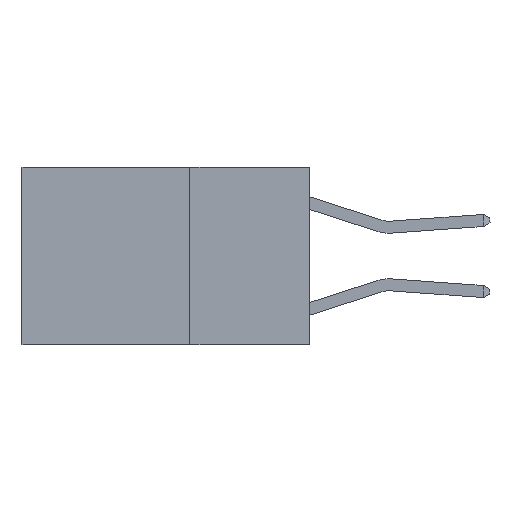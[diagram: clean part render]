
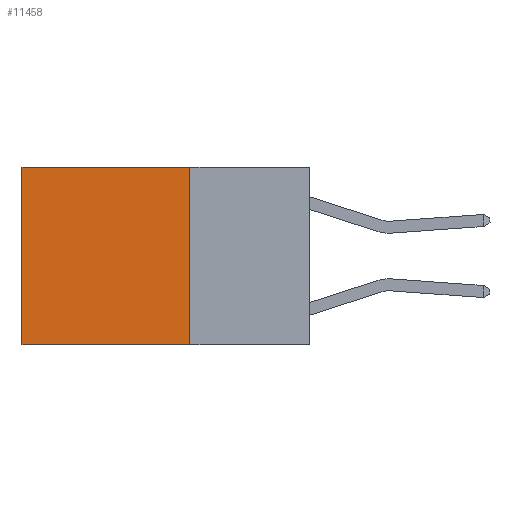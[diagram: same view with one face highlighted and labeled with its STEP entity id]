
A CAD part, left-side view. The second image highlights one B-rep face of the part: STEP entity #11458.
In plain terms, the highlighted planar face has unit normal (-1, 0, 0).
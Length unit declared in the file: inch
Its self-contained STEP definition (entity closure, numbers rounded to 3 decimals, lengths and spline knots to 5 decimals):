
#549 = DIRECTION ( 'NONE',  ( 0., 0., -1. ) ) ;
#1560 = VECTOR ( 'NONE', #18103, 39.37008 ) ;
#1615 = VERTEX_POINT ( 'NONE', #12100 ) ;
#2018 = EDGE_CURVE ( 'NONE', #11484, #3842, #4054, .T. ) ;
#2330 = LINE ( 'NONE', #20022, #9081 ) ;
#3172 = ORIENTED_EDGE ( 'NONE', *, *, #21066, .T. ) ;
#3365 = CARTESIAN_POINT ( 'NONE',  ( 0.2625, 0.25, 0. ) ) ;
#3842 = VERTEX_POINT ( 'NONE', #13780 ) ;
#4054 = LINE ( 'NONE', #11762, #20720 ) ;
#4917 = CARTESIAN_POINT ( 'NONE',  ( 0.2625, 0.25, 0. ) ) ;
#6574 = DIRECTION ( 'NONE',  ( 0., 0., -1. ) ) ;
#6920 = CARTESIAN_POINT ( 'NONE',  ( 0.2625, 0.25, 0. ) ) ;
#6943 = EDGE_CURVE ( 'NONE', #16107, #1615, #12388, .T. ) ;
#7132 = DIRECTION ( 'NONE',  ( 1., 0., 0. ) ) ;
#8471 = DIRECTION ( 'NONE',  ( 0., 1., 0. ) ) ;
#9081 = VECTOR ( 'NONE', #8471, 39.37008 ) ;
#9291 = ORIENTED_EDGE ( 'NONE', *, *, #18283, .F. ) ;
#11098 = VECTOR ( 'NONE', #6574, 39.37008 ) ;
#11458 = ADVANCED_FACE ( 'NONE', ( #20952 ), #16909, .F. ) ;
#11484 = VERTEX_POINT ( 'NONE', #15468 ) ;
#11762 = CARTESIAN_POINT ( 'NONE',  ( 0.2625, 0.6, 0. ) ) ;
#12100 = CARTESIAN_POINT ( 'NONE',  ( 0.2625, 0.25, -0.37 ) ) ;
#12388 = LINE ( 'NONE', #4917, #11098 ) ;
#13756 = ORIENTED_EDGE ( 'NONE', *, *, #6943, .F. ) ;
#13780 = CARTESIAN_POINT ( 'NONE',  ( 0.2625, 0.6, -0.37 ) ) ;
#14736 = LINE ( 'NONE', #14924, #1560 ) ;
#14924 = CARTESIAN_POINT ( 'NONE',  ( 0.2625, 0.25, 0. ) ) ;
#15267 = AXIS2_PLACEMENT_3D ( 'NONE', #6920, #7132, #549 ) ;
#15378 = ORIENTED_EDGE ( 'NONE', *, *, #2018, .T. ) ;
#15468 = CARTESIAN_POINT ( 'NONE',  ( 0.2625, 0.6, 0. ) ) ;
#16107 = VERTEX_POINT ( 'NONE', #3365 ) ;
#16909 = PLANE ( 'NONE',  #15267 ) ;
#18007 = EDGE_LOOP ( 'NONE', ( #15378, #9291, #13756, #3172 ) ) ;
#18103 = DIRECTION ( 'NONE',  ( 0., 1., 0. ) ) ;
#18283 = EDGE_CURVE ( 'NONE', #1615, #3842, #2330, .T. ) ;
#18935 = DIRECTION ( 'NONE',  ( 0., 0., -1. ) ) ;
#20022 = CARTESIAN_POINT ( 'NONE',  ( 0.2625, 0.25, -0.37 ) ) ;
#20720 = VECTOR ( 'NONE', #18935, 39.37008 ) ;
#20952 = FACE_OUTER_BOUND ( 'NONE', #18007, .T. ) ;
#21066 = EDGE_CURVE ( 'NONE', #16107, #11484, #14736, .T. ) ;
